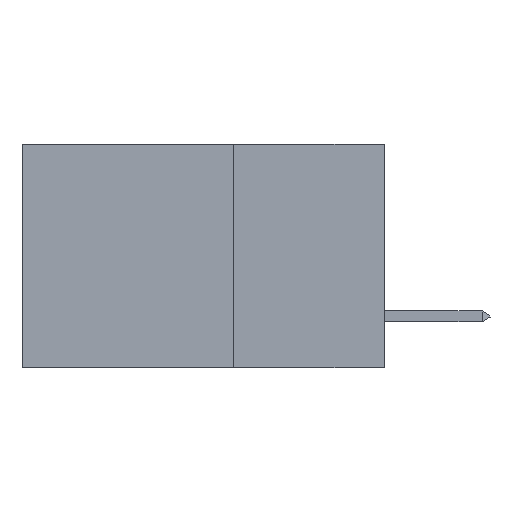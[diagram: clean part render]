
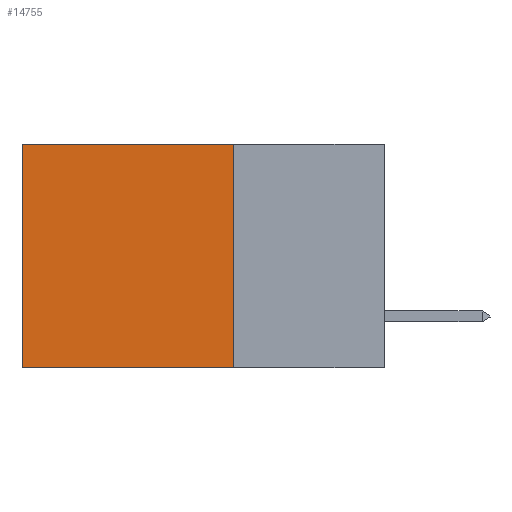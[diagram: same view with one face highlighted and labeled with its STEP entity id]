
A CAD part, left-side view. The second image highlights one B-rep face of the part: STEP entity #14755.
In plain terms, the highlighted planar face has unit normal (-1, 0, 0).
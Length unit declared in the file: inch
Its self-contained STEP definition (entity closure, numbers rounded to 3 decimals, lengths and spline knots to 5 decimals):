
#454 = EDGE_CURVE ( 'NONE', #12883, #6720, #7425, .T. ) ;
#1448 = VECTOR ( 'NONE', #9576, 39.37008 ) ;
#1812 = CARTESIAN_POINT ( 'NONE',  ( 0.2875, 0.6, 0. ) ) ;
#1869 = CARTESIAN_POINT ( 'NONE',  ( 0.2875, 0.6, 0. ) ) ;
#2243 = DIRECTION ( 'NONE',  ( 1., 0., 0. ) ) ;
#2360 = CARTESIAN_POINT ( 'NONE',  ( 0.2875, 0.25, 0. ) ) ;
#2430 = CARTESIAN_POINT ( 'NONE',  ( 0.2875, 0.25, -0.37 ) ) ;
#2739 = FACE_OUTER_BOUND ( 'NONE', #15645, .T. ) ;
#3492 = EDGE_CURVE ( 'NONE', #12883, #3757, #4875, .T. ) ;
#3757 = VERTEX_POINT ( 'NONE', #2430 ) ;
#4380 = ORIENTED_EDGE ( 'NONE', *, *, #3492, .F. ) ;
#4532 = VERTEX_POINT ( 'NONE', #11295 ) ;
#4823 = CARTESIAN_POINT ( 'NONE',  ( 0.2875, 0.25, 0. ) ) ;
#4875 = LINE ( 'NONE', #8310, #1448 ) ;
#5373 = ORIENTED_EDGE ( 'NONE', *, *, #13836, .T. ) ;
#6501 = LINE ( 'NONE', #9043, #7947 ) ;
#6720 = VERTEX_POINT ( 'NONE', #1812 ) ;
#7240 = ORIENTED_EDGE ( 'NONE', *, *, #9500, .F. ) ;
#7425 = LINE ( 'NONE', #4823, #11933 ) ;
#7450 = PLANE ( 'NONE',  #12391 ) ;
#7480 = DIRECTION ( 'NONE',  ( 0., 1., 0. ) ) ;
#7947 = VECTOR ( 'NONE', #16734, 39.37008 ) ;
#8310 = CARTESIAN_POINT ( 'NONE',  ( 0.2875, 0.25, 0. ) ) ;
#9043 = CARTESIAN_POINT ( 'NONE',  ( 0.2875, 0.25, -0.37 ) ) ;
#9094 = VECTOR ( 'NONE', #14920, 39.37008 ) ;
#9500 = EDGE_CURVE ( 'NONE', #3757, #4532, #6501, .T. ) ;
#9576 = DIRECTION ( 'NONE',  ( 0., 0., -1. ) ) ;
#11295 = CARTESIAN_POINT ( 'NONE',  ( 0.2875, 0.6, -0.37 ) ) ;
#11933 = VECTOR ( 'NONE', #7480, 39.37008 ) ;
#12391 = AXIS2_PLACEMENT_3D ( 'NONE', #2360, #2243, #16439 ) ;
#12795 = LINE ( 'NONE', #1869, #9094 ) ;
#12883 = VERTEX_POINT ( 'NONE', #15217 ) ;
#12964 = ORIENTED_EDGE ( 'NONE', *, *, #454, .T. ) ;
#13836 = EDGE_CURVE ( 'NONE', #6720, #4532, #12795, .T. ) ;
#14755 = ADVANCED_FACE ( 'NONE', ( #2739 ), #7450, .F. ) ;
#14920 = DIRECTION ( 'NONE',  ( 0., 0., -1. ) ) ;
#15217 = CARTESIAN_POINT ( 'NONE',  ( 0.2875, 0.25, 0. ) ) ;
#15645 = EDGE_LOOP ( 'NONE', ( #5373, #7240, #4380, #12964 ) ) ;
#16439 = DIRECTION ( 'NONE',  ( 0., 0., -1. ) ) ;
#16734 = DIRECTION ( 'NONE',  ( 0., 1., 0. ) ) ;
